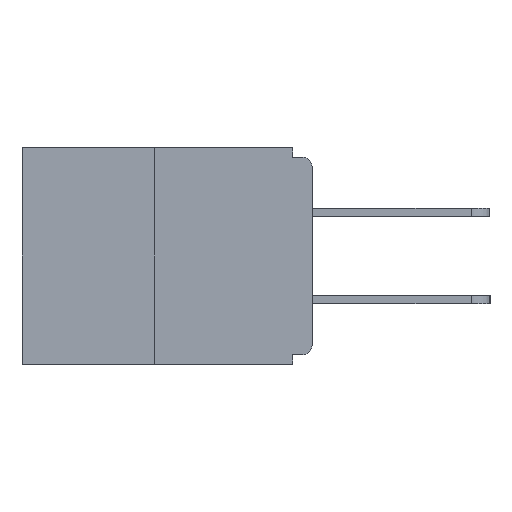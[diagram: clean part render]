
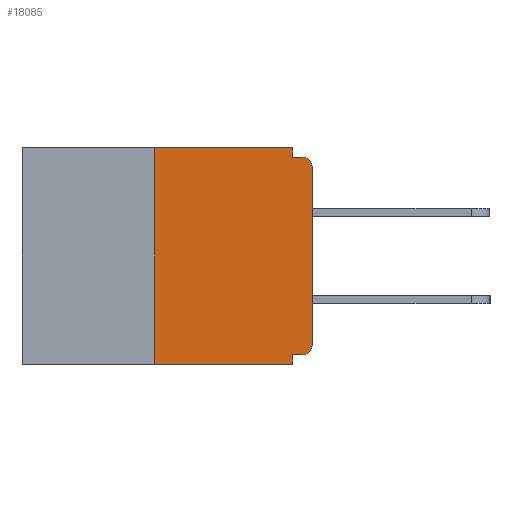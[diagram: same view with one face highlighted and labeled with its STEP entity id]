
A CAD part, left-side view. The second image highlights one B-rep face of the part: STEP entity #18085.
In plain terms, the highlighted planar face has unit normal (-1, 0, 0).
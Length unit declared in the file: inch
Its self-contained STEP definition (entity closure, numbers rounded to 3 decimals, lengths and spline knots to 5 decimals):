
#462 = VERTEX_POINT ( 'NONE', #5788 ) ;
#469 = VECTOR ( 'NONE', #4712, 39.37008 ) ;
#698 = CARTESIAN_POINT ( 'NONE',  ( 0., 0.031, 0. ) ) ;
#708 = EDGE_CURVE ( 'NONE', #7802, #15730, #5569, .T. ) ;
#935 = DIRECTION ( 'NONE',  ( 0., 0., -1. ) ) ;
#955 = CARTESIAN_POINT ( 'NONE',  ( 0., 0.031, -0.343 ) ) ;
#1054 = EDGE_CURVE ( 'NONE', #13387, #1981, #6186, .T. ) ;
#1352 = CARTESIAN_POINT ( 'NONE',  ( 0., 0.031, -0.343 ) ) ;
#1528 = DIRECTION ( 'NONE',  ( 0., 1., 0. ) ) ;
#1967 = CARTESIAN_POINT ( 'NONE',  ( 0., 0.25, -0.343 ) ) ;
#1981 = VERTEX_POINT ( 'NONE', #13492 ) ;
#2083 = CARTESIAN_POINT ( 'NONE',  ( 0., 0.031, 0. ) ) ;
#2106 = ORIENTED_EDGE ( 'NONE', *, *, #17156, .F. ) ;
#2181 = PLANE ( 'NONE',  #15764 ) ;
#2461 = ORIENTED_EDGE ( 'NONE', *, *, #1054, .T. ) ;
#2947 = DIRECTION ( 'NONE',  ( 0., -1., 0. ) ) ;
#3142 = DIRECTION ( 'NONE',  ( 0., -1., 0. ) ) ;
#4081 = EDGE_CURVE ( 'NONE', #15730, #462, #18306, .T. ) ;
#4636 = EDGE_LOOP ( 'NONE', ( #14610, #6679, #12472, #13268, #2106, #2461, #10343, #18349, #19445, #6402 ) ) ;
#4712 = DIRECTION ( 'NONE',  ( 0., -1., 0. ) ) ;
#4739 = DIRECTION ( 'NONE',  ( -1., 0., 0. ) ) ;
#5045 = CARTESIAN_POINT ( 'NONE',  ( 0., 0.031, -0.328 ) ) ;
#5236 = EDGE_CURVE ( 'NONE', #11194, #15397, #19453, .T. ) ;
#5418 = VECTOR ( 'NONE', #1528, 39.37008 ) ;
#5569 = LINE ( 'NONE', #698, #8051 ) ;
#5665 = DIRECTION ( 'NONE',  ( 0., 0., -1. ) ) ;
#5744 = AXIS2_PLACEMENT_3D ( 'NONE', #15997, #8627, #935 ) ;
#5788 = CARTESIAN_POINT ( 'NONE',  ( 0., 0.015, -0.015 ) ) ;
#6003 = DIRECTION ( 'NONE',  ( 0., 0., 1. ) ) ;
#6186 = CIRCLE ( 'NONE', #14248, 0.015 ) ;
#6402 = ORIENTED_EDGE ( 'NONE', *, *, #708, .F. ) ;
#6420 = VECTOR ( 'NONE', #7136, 39.37008 ) ;
#6679 = ORIENTED_EDGE ( 'NONE', *, *, #7417, .F. ) ;
#6975 = VECTOR ( 'NONE', #6003, 39.37008 ) ;
#7136 = DIRECTION ( 'NONE',  ( 0., 0., -1. ) ) ;
#7329 = LINE ( 'NONE', #10661, #6975 ) ;
#7417 = EDGE_CURVE ( 'NONE', #8226, #8827, #12313, .T. ) ;
#7802 = VERTEX_POINT ( 'NONE', #2083 ) ;
#7961 = FACE_OUTER_BOUND ( 'NONE', #4636, .T. ) ;
#8051 = VECTOR ( 'NONE', #5665, 39.37008 ) ;
#8226 = VERTEX_POINT ( 'NONE', #1967 ) ;
#8335 = VECTOR ( 'NONE', #3142, 39.37008 ) ;
#8627 = DIRECTION ( 'NONE',  ( -1., 0., 0. ) ) ;
#8633 = CIRCLE ( 'NONE', #5744, 0.015 ) ;
#8690 = VECTOR ( 'NONE', #2947, 39.37008 ) ;
#8817 = VECTOR ( 'NONE', #18473, 39.37008 ) ;
#8827 = VERTEX_POINT ( 'NONE', #11448 ) ;
#9166 = LINE ( 'NONE', #15535, #469 ) ;
#9386 = EDGE_CURVE ( 'NONE', #8827, #7802, #9166, .T. ) ;
#9575 = DIRECTION ( 'NONE',  ( 1., 0., 0. ) ) ;
#9677 = DIRECTION ( 'NONE',  ( 0., 0., -1. ) ) ;
#9945 = CARTESIAN_POINT ( 'NONE',  ( 0., 0., -0.03 ) ) ;
#10343 = ORIENTED_EDGE ( 'NONE', *, *, #15513, .T. ) ;
#10539 = EDGE_CURVE ( 'NONE', #8226, #15397, #10634, .T. ) ;
#10634 = LINE ( 'NONE', #19921, #8335 ) ;
#10661 = CARTESIAN_POINT ( 'NONE',  ( 0., 0., 0. ) ) ;
#11194 = VERTEX_POINT ( 'NONE', #5045 ) ;
#11448 = CARTESIAN_POINT ( 'NONE',  ( 0., 0.25, 0. ) ) ;
#11740 = CARTESIAN_POINT ( 'NONE',  ( 0., 0.031, -0.015 ) ) ;
#12313 = LINE ( 'NONE', #14759, #8817 ) ;
#12472 = ORIENTED_EDGE ( 'NONE', *, *, #10539, .T. ) ;
#13268 = ORIENTED_EDGE ( 'NONE', *, *, #5236, .F. ) ;
#13387 = VERTEX_POINT ( 'NONE', #16106 ) ;
#13492 = CARTESIAN_POINT ( 'NONE',  ( 0., 0., -0.313 ) ) ;
#14229 = DIRECTION ( 'NONE',  ( 0., 0., -1. ) ) ;
#14248 = AXIS2_PLACEMENT_3D ( 'NONE', #18485, #4739, #14229 ) ;
#14610 = ORIENTED_EDGE ( 'NONE', *, *, #9386, .F. ) ;
#14759 = CARTESIAN_POINT ( 'NONE',  ( 0., 0.25, 0. ) ) ;
#15378 = CARTESIAN_POINT ( 'NONE',  ( 0., 0., -0.015 ) ) ;
#15397 = VERTEX_POINT ( 'NONE', #1352 ) ;
#15513 = EDGE_CURVE ( 'NONE', #1981, #18628, #7329, .T. ) ;
#15535 = CARTESIAN_POINT ( 'NONE',  ( 0., 0.46, 0. ) ) ;
#15730 = VERTEX_POINT ( 'NONE', #11740 ) ;
#15764 = AXIS2_PLACEMENT_3D ( 'NONE', #17551, #9575, #9677 ) ;
#15997 = CARTESIAN_POINT ( 'NONE',  ( 0., 0.015, -0.03 ) ) ;
#16106 = CARTESIAN_POINT ( 'NONE',  ( 0., 0.015, -0.328 ) ) ;
#16506 = CARTESIAN_POINT ( 'NONE',  ( 0., 0., -0.328 ) ) ;
#17099 = EDGE_CURVE ( 'NONE', #18628, #462, #8633, .T. ) ;
#17156 = EDGE_CURVE ( 'NONE', #13387, #11194, #18219, .T. ) ;
#17551 = CARTESIAN_POINT ( 'NONE',  ( 0., 0.46, 0. ) ) ;
#18085 = ADVANCED_FACE ( 'NONE', ( #7961 ), #2181, .F. ) ;
#18219 = LINE ( 'NONE', #16506, #5418 ) ;
#18306 = LINE ( 'NONE', #15378, #8690 ) ;
#18349 = ORIENTED_EDGE ( 'NONE', *, *, #17099, .T. ) ;
#18473 = DIRECTION ( 'NONE',  ( 0., 0., 1. ) ) ;
#18485 = CARTESIAN_POINT ( 'NONE',  ( 0., 0.015, -0.313 ) ) ;
#18628 = VERTEX_POINT ( 'NONE', #9945 ) ;
#19445 = ORIENTED_EDGE ( 'NONE', *, *, #4081, .F. ) ;
#19453 = LINE ( 'NONE', #955, #6420 ) ;
#19921 = CARTESIAN_POINT ( 'NONE',  ( 0., 0.46, -0.343 ) ) ;
